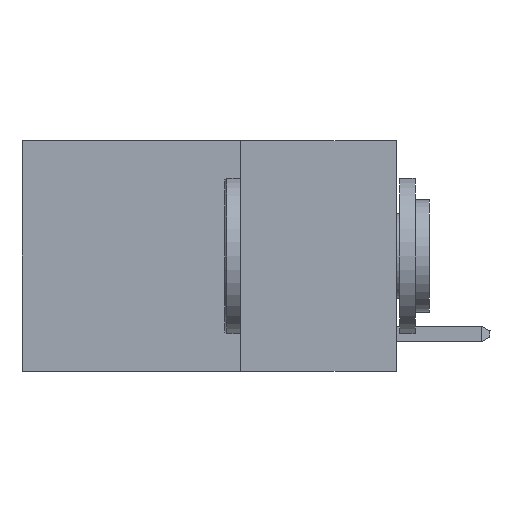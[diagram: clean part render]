
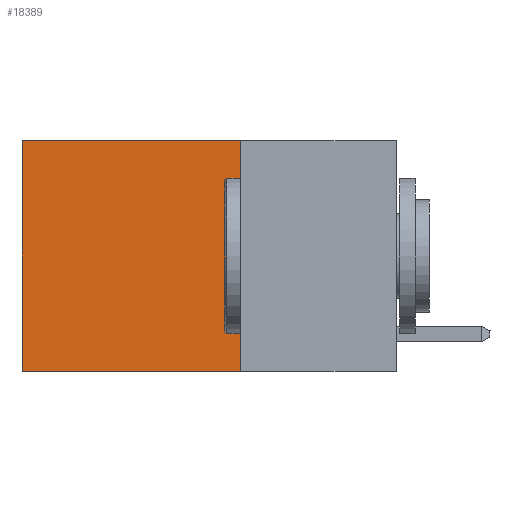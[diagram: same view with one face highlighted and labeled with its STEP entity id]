
A CAD part, left-side view. The second image highlights one B-rep face of the part: STEP entity #18389.
In plain terms, the highlighted planar face has unit normal (-1, 0, 0).
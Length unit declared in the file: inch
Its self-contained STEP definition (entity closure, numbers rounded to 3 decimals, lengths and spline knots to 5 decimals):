
#2199 = DIRECTION ( 'NONE',  ( 0., 1., 0. ) ) ;
#2933 = LINE ( 'NONE', #15717, #11108 ) ;
#3857 = CARTESIAN_POINT ( 'NONE',  ( 0.2625, 0.25, 0. ) ) ;
#4245 = VECTOR ( 'NONE', #2199, 39.37008 ) ;
#4472 = DIRECTION ( 'NONE',  ( 0., 1., 0. ) ) ;
#4514 = CARTESIAN_POINT ( 'NONE',  ( 0.2625, 0.25, 0. ) ) ;
#5187 = DIRECTION ( 'NONE',  ( 1., 0., 0. ) ) ;
#5283 = ORIENTED_EDGE ( 'NONE', *, *, #5299, .T. ) ;
#5299 = EDGE_CURVE ( 'NONE', #19158, #5748, #7005, .T. ) ;
#5374 = CARTESIAN_POINT ( 'NONE',  ( 0.2625, 0.6, 0. ) ) ;
#5748 = VERTEX_POINT ( 'NONE', #19782 ) ;
#6666 = ORIENTED_EDGE ( 'NONE', *, *, #15418, .F. ) ;
#7005 = LINE ( 'NONE', #17938, #10644 ) ;
#7134 = CARTESIAN_POINT ( 'NONE',  ( 0.2625, 0.25, -0.37 ) ) ;
#7218 = VERTEX_POINT ( 'NONE', #19402 ) ;
#7642 = ORIENTED_EDGE ( 'NONE', *, *, #10871, .F. ) ;
#8080 = FACE_OUTER_BOUND ( 'NONE', #14642, .T. ) ;
#8278 = PLANE ( 'NONE',  #16137 ) ;
#8813 = ORIENTED_EDGE ( 'NONE', *, *, #14055, .T. ) ;
#10644 = VECTOR ( 'NONE', #19190, 39.37008 ) ;
#10871 = EDGE_CURVE ( 'NONE', #11834, #7218, #18822, .T. ) ;
#11108 = VECTOR ( 'NONE', #4472, 39.37008 ) ;
#11834 = VERTEX_POINT ( 'NONE', #4514 ) ;
#14055 = EDGE_CURVE ( 'NONE', #11834, #19158, #2933, .T. ) ;
#14179 = DIRECTION ( 'NONE',  ( 0., 0., -1. ) ) ;
#14642 = EDGE_LOOP ( 'NONE', ( #5283, #6666, #7642, #8813 ) ) ;
#14968 = LINE ( 'NONE', #7134, #4245 ) ;
#15418 = EDGE_CURVE ( 'NONE', #7218, #5748, #14968, .T. ) ;
#15717 = CARTESIAN_POINT ( 'NONE',  ( 0.2625, 0.25, 0. ) ) ;
#16137 = AXIS2_PLACEMENT_3D ( 'NONE', #3857, #5187, #17565 ) ;
#16615 = VECTOR ( 'NONE', #14179, 39.37008 ) ;
#17565 = DIRECTION ( 'NONE',  ( 0., 0., -1. ) ) ;
#17938 = CARTESIAN_POINT ( 'NONE',  ( 0.2625, 0.6, 0. ) ) ;
#18389 = ADVANCED_FACE ( 'NONE', ( #8080 ), #8278, .F. ) ;
#18822 = LINE ( 'NONE', #20273, #16615 ) ;
#19158 = VERTEX_POINT ( 'NONE', #5374 ) ;
#19190 = DIRECTION ( 'NONE',  ( 0., 0., -1. ) ) ;
#19402 = CARTESIAN_POINT ( 'NONE',  ( 0.2625, 0.25, -0.37 ) ) ;
#19782 = CARTESIAN_POINT ( 'NONE',  ( 0.2625, 0.6, -0.37 ) ) ;
#20273 = CARTESIAN_POINT ( 'NONE',  ( 0.2625, 0.25, 0. ) ) ;
